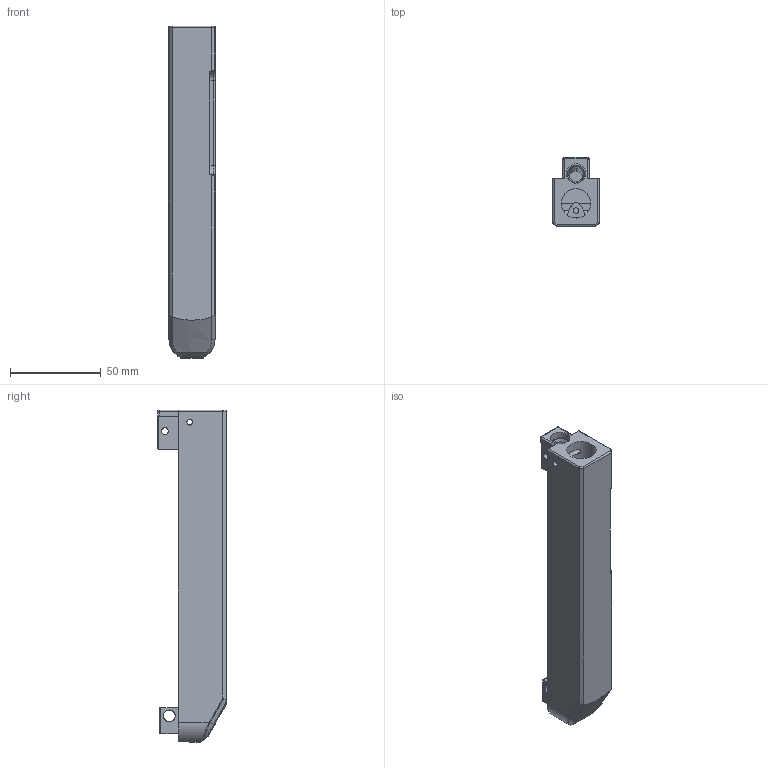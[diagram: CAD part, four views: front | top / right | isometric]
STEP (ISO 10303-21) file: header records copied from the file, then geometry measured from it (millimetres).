
FILE_DESCRIPTION (( 'STEP AP214' ), '1' );
FILE_NAME ('Merlin 60 release no rail.STEP', '2021-07-15T18:08:44', ( 'RJ' ), ( '' ), 'SwSTEP 2.0', 'SolidWorks 2015', '' );
FILE_SCHEMA (( 'AUTOMOTIVE_DESIGN' ));
Length unit declared in the file: millimetre
Products named in the file (1): Merlin 60 release no rail
Bounding box: 25.5 x 38 x 183 mm (x, y, z)
Volume: 55455.7 mm3; surface area: 28167.5 mm2
Topology: 1 solids, 1 shells, 136 faces, 358 edges, 225 vertices
Faces by surface type: plane 54, cylinder 52, bspline 26, torus 4
Entity records: 6239 total; most frequent: CARTESIAN_POINT 3067, ORIENTED_EDGE 716, DIRECTION 551, EDGE_CURVE 358, VERTEX_POINT 225, LINE 197, VECTOR 197, AXIS2_PLACEMENT_3D 177
